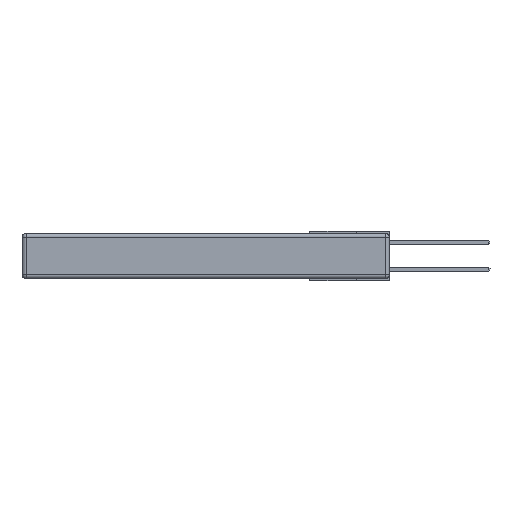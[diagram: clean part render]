
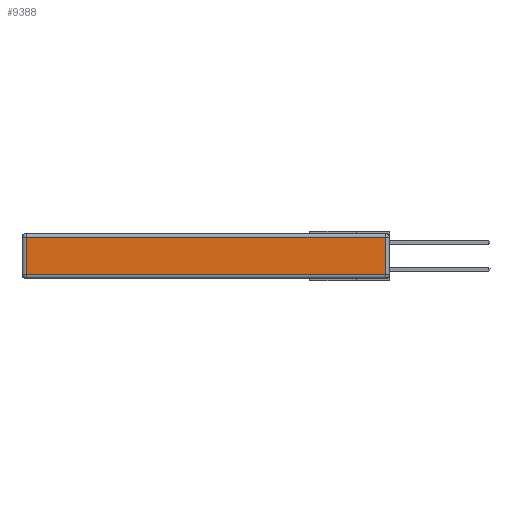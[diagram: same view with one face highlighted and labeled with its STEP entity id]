
A CAD part, left-side view. The second image highlights one B-rep face of the part: STEP entity #9388.
In plain terms, the highlighted planar face has unit normal (-1, 0, 0).
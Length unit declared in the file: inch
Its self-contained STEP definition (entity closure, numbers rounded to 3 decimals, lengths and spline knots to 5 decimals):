
#2893 = EDGE_CURVE ( 'NONE', #7390, #5850, #9402, .T. ) ;
#5674 = CARTESIAN_POINT ( 'NONE',  ( 0., 0., -0.313 ) ) ;
#5850 = VERTEX_POINT ( 'NONE', #26279 ) ;
#6306 = PLANE ( 'NONE',  #25599 ) ;
#7381 = EDGE_CURVE ( 'NONE', #5850, #13677, #18927, .T. ) ;
#7390 = VERTEX_POINT ( 'NONE', #9692 ) ;
#7696 = VECTOR ( 'NONE', #18919, 39.37008 ) ;
#8371 = LINE ( 'NONE', #12559, #7696 ) ;
#8375 = CARTESIAN_POINT ( 'NONE',  ( 0., 0., -0.343 ) ) ;
#9388 = ADVANCED_FACE ( 'NONE', ( #26784 ), #6306, .T. ) ;
#9402 = LINE ( 'NONE', #15305, #22953 ) ;
#9692 = CARTESIAN_POINT ( 'NONE',  ( 0., 2.72, -0.03 ) ) ;
#10520 = DIRECTION ( 'NONE',  ( -1., 0., 0. ) ) ;
#10907 = ORIENTED_EDGE ( 'NONE', *, *, #2893, .T. ) ;
#12088 = DIRECTION ( 'NONE',  ( 0., -1., 0. ) ) ;
#12559 = CARTESIAN_POINT ( 'NONE',  ( 0., 2.75, -0.03 ) ) ;
#13367 = DIRECTION ( 'NONE',  ( 0., 0., -1. ) ) ;
#13641 = EDGE_CURVE ( 'NONE', #19033, #7390, #8371, .T. ) ;
#13677 = VERTEX_POINT ( 'NONE', #14849 ) ;
#14849 = CARTESIAN_POINT ( 'NONE',  ( 0., 0.03, -0.313 ) ) ;
#15211 = LINE ( 'NONE', #24768, #24118 ) ;
#15305 = CARTESIAN_POINT ( 'NONE',  ( 0., 2.72, -0.343 ) ) ;
#16590 = ORIENTED_EDGE ( 'NONE', *, *, #7381, .T. ) ;
#17717 = EDGE_LOOP ( 'NONE', ( #16590, #21434, #22165, #10907 ) ) ;
#18919 = DIRECTION ( 'NONE',  ( 0., 1., 0. ) ) ;
#18927 = LINE ( 'NONE', #5674, #23873 ) ;
#19033 = VERTEX_POINT ( 'NONE', #20302 ) ;
#20302 = CARTESIAN_POINT ( 'NONE',  ( 0., 0.03, -0.03 ) ) ;
#21208 = EDGE_CURVE ( 'NONE', #13677, #19033, #15211, .T. ) ;
#21434 = ORIENTED_EDGE ( 'NONE', *, *, #21208, .T. ) ;
#22165 = ORIENTED_EDGE ( 'NONE', *, *, #13641, .T. ) ;
#22953 = VECTOR ( 'NONE', #13367, 39.37008 ) ;
#23873 = VECTOR ( 'NONE', #12088, 39.37008 ) ;
#24118 = VECTOR ( 'NONE', #24486, 39.37008 ) ;
#24486 = DIRECTION ( 'NONE',  ( 0., 0., 1. ) ) ;
#24768 = CARTESIAN_POINT ( 'NONE',  ( 0., 0.03, -0.343 ) ) ;
#25268 = DIRECTION ( 'NONE',  ( 0., 0., 1. ) ) ;
#25599 = AXIS2_PLACEMENT_3D ( 'NONE', #8375, #10520, #25268 ) ;
#26279 = CARTESIAN_POINT ( 'NONE',  ( 0., 2.72, -0.313 ) ) ;
#26784 = FACE_OUTER_BOUND ( 'NONE', #17717, .T. ) ;
